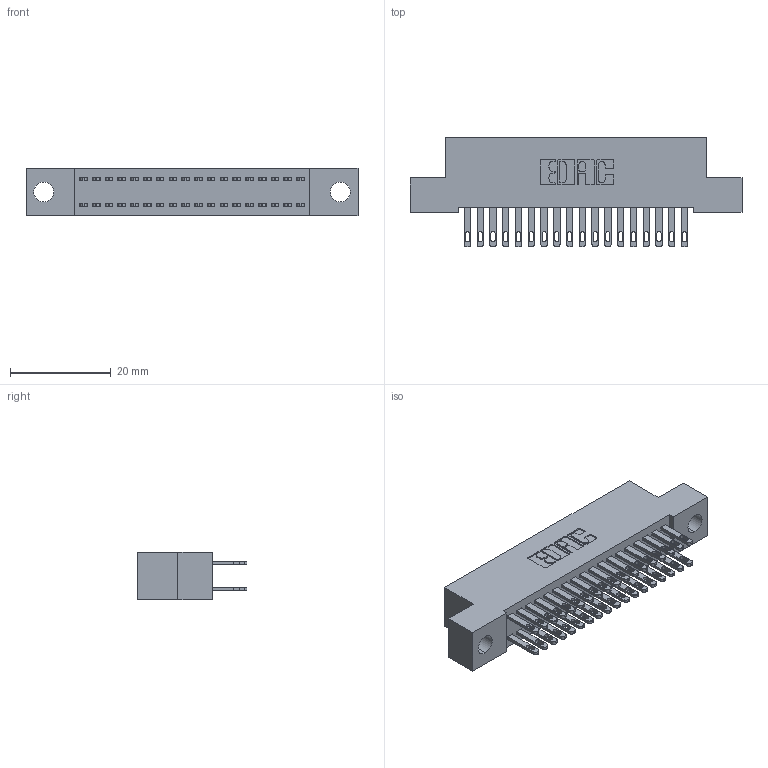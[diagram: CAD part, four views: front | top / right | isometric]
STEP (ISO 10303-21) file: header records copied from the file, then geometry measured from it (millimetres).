
FILE_DESCRIPTION (( 'STEP AP203' ), '1' );
FILE_NAME ('892-036-500-204.STEP', '2020-09-21T15:57:00', ( '' ), ( '' ), 'SwSTEP 2.0', 'SolidWorks 2020', '' );
FILE_SCHEMA (( 'CONFIG_CONTROL_DESIGN' ));
Length unit declared in the file: inch
Products named in the file (3): 892-036-500-204; 842 Part_.156 TH; 345-292-001_345-293-100
Assembly tree (37 placements, depth 2):
  892-036-500-204
    842 Part_.156 TH
    345-292-001_345-293-100  x36
Bounding box: 66.04 x 21.85 x 9.4 mm (x, y, z)
Volume: 5843.1 mm3; surface area: 9088.6 mm2
Topology: 37 solids, 37 shells, 1838 faces, 5591 edges, 3726 vertices
Faces by surface type: plane 1146, cylinder 692
Entity records: 14485 total; most frequent: CARTESIAN_POINT 2426, ORIENTED_EDGE 2362, DIRECTION 2117, EDGE_CURVE 1181, VECTOR 1049, LINE 1049, VERTEX_POINT 786, AXIS2_PLACEMENT_3D 534
